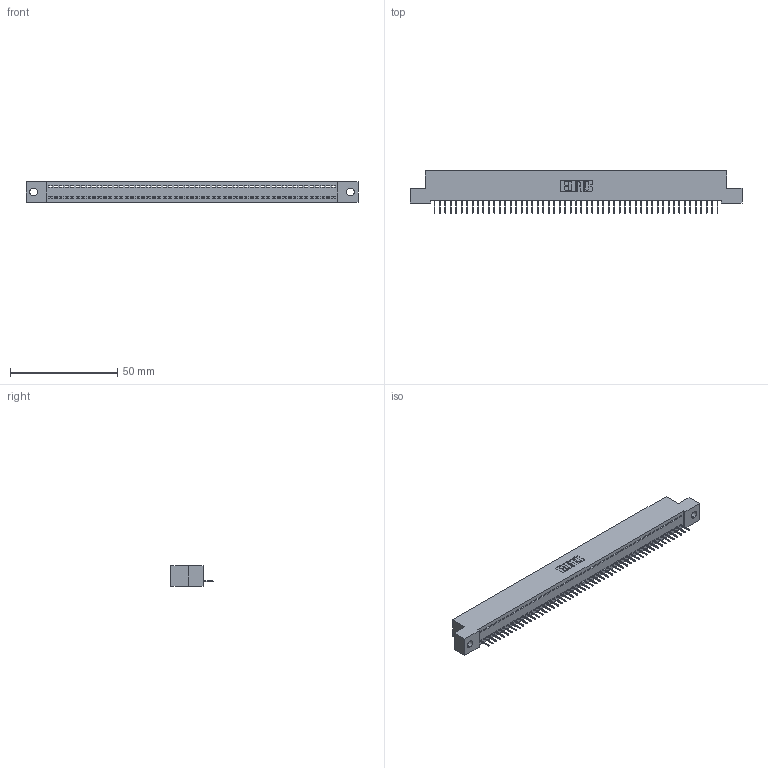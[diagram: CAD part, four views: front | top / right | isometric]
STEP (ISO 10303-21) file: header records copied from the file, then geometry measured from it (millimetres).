
FILE_DESCRIPTION (( 'STEP AP203' ), '1' );
FILE_NAME ('342-053-524-102.STEP', '2019-10-03T02:11:09', ( '' ), ( '' ), 'SwSTEP 2.0', 'SolidWorks 2016', '' );
FILE_SCHEMA (( 'CONFIG_CONTROL_DESIGN' ));
Length unit declared in the file: inch
Products named in the file (3): 342 Part_.128 Slot; 345-292-001_345-293-124; 342-053-524-102
Assembly tree (54 placements, depth 2):
  342-053-524-102
    342 Part_.128 Slot
    345-292-001_345-293-124  x53
Bounding box: 154.94 x 19.69 x 9.4 mm (x, y, z)
Volume: 13364.2 mm3; surface area: 18939.3 mm2
Topology: 54 solids, 54 shells, 3400 faces, 9851 edges, 6354 vertices
Faces by surface type: plane 2614, cylinder 786
Entity records: 31055 total; most frequent: CARTESIAN_POINT 5361, ORIENTED_EDGE 5350, DIRECTION 4501, EDGE_CURVE 2675, LINE 2551, VECTOR 2551, VERTEX_POINT 1778, AXIS2_PLACEMENT_3D 975
